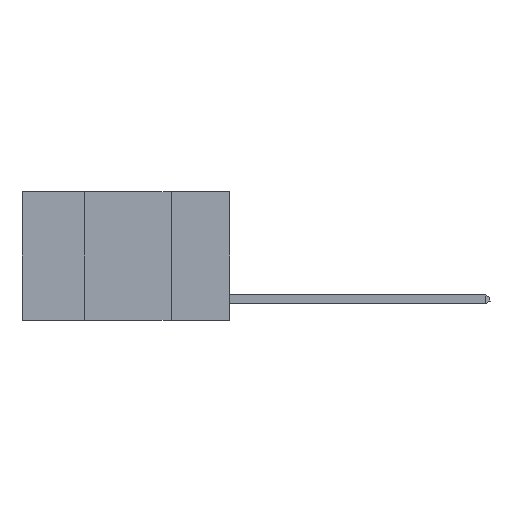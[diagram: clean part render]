
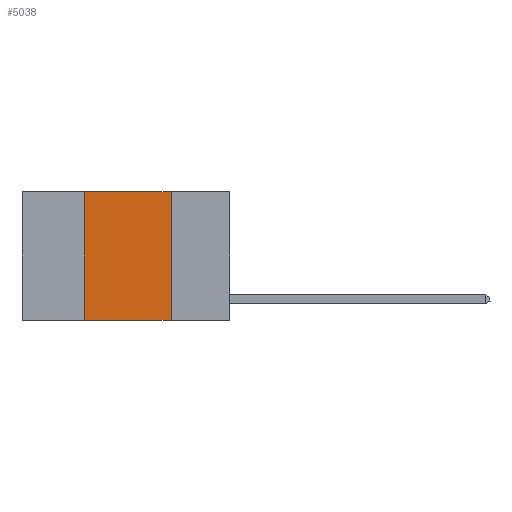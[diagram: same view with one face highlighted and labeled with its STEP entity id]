
A CAD part, left-side view. The second image highlights one B-rep face of the part: STEP entity #5038.
In plain terms, the highlighted planar face has unit normal (-1, 0, 0).
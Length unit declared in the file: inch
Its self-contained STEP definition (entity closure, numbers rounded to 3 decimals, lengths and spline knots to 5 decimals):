
#378 = VERTEX_POINT ( 'NONE', #5244 ) ;
#423 = ORIENTED_EDGE ( 'NONE', *, *, #6462, .T. ) ;
#684 = CARTESIAN_POINT ( 'NONE',  ( 0., 0.6, 0. ) ) ;
#1729 = DIRECTION ( 'NONE',  ( 0., -1., 0. ) ) ;
#1814 = VECTOR ( 'NONE', #1729, 39.37008 ) ;
#1910 = DIRECTION ( 'NONE',  ( 0., 0., 1. ) ) ;
#2093 = ORIENTED_EDGE ( 'NONE', *, *, #7032, .F. ) ;
#2151 = DIRECTION ( 'NONE',  ( 1., 0., 0. ) ) ;
#2262 = VECTOR ( 'NONE', #6485, 39.37008 ) ;
#2380 = VERTEX_POINT ( 'NONE', #6818 ) ;
#3168 = CARTESIAN_POINT ( 'NONE',  ( 0., 0.17, 0. ) ) ;
#3298 = VERTEX_POINT ( 'NONE', #3308 ) ;
#3308 = CARTESIAN_POINT ( 'NONE',  ( 0., 0.17, 0. ) ) ;
#3408 = LINE ( 'NONE', #6216, #5043 ) ;
#3739 = LINE ( 'NONE', #7967, #1814 ) ;
#4129 = AXIS2_PLACEMENT_3D ( 'NONE', #684, #2151, #6921 ) ;
#4440 = EDGE_CURVE ( 'NONE', #3298, #2380, #8612, .T. ) ;
#4628 = ORIENTED_EDGE ( 'NONE', *, *, #5743, .F. ) ;
#4888 = PLANE ( 'NONE',  #4129 ) ;
#4989 = CARTESIAN_POINT ( 'NONE',  ( 0., 0.6, 0. ) ) ;
#5038 = ADVANCED_FACE ( 'NONE', ( #7009 ), #4888, .F. ) ;
#5043 = VECTOR ( 'NONE', #1910, 39.37008 ) ;
#5132 = DIRECTION ( 'NONE',  ( 0., 0., -1. ) ) ;
#5244 = CARTESIAN_POINT ( 'NONE',  ( 0., 0.42, -0.37 ) ) ;
#5571 = ORIENTED_EDGE ( 'NONE', *, *, #4440, .F. ) ;
#5743 = EDGE_CURVE ( 'NONE', #7724, #3298, #6444, .T. ) ;
#6170 = VECTOR ( 'NONE', #5132, 39.37008 ) ;
#6216 = CARTESIAN_POINT ( 'NONE',  ( 0., 0.42, 0. ) ) ;
#6444 = LINE ( 'NONE', #4989, #2262 ) ;
#6462 = EDGE_CURVE ( 'NONE', #378, #2380, #3739, .T. ) ;
#6485 = DIRECTION ( 'NONE',  ( 0., -1., 0. ) ) ;
#6818 = CARTESIAN_POINT ( 'NONE',  ( 0., 0.17, -0.37 ) ) ;
#6921 = DIRECTION ( 'NONE',  ( 0., 0., -1. ) ) ;
#6966 = EDGE_LOOP ( 'NONE', ( #5571, #4628, #2093, #423 ) ) ;
#7009 = FACE_OUTER_BOUND ( 'NONE', #6966, .T. ) ;
#7032 = EDGE_CURVE ( 'NONE', #378, #7724, #3408, .T. ) ;
#7724 = VERTEX_POINT ( 'NONE', #9000 ) ;
#7967 = CARTESIAN_POINT ( 'NONE',  ( 0., 0.6, -0.37 ) ) ;
#8612 = LINE ( 'NONE', #3168, #6170 ) ;
#9000 = CARTESIAN_POINT ( 'NONE',  ( 0., 0.42, 0. ) ) ;
